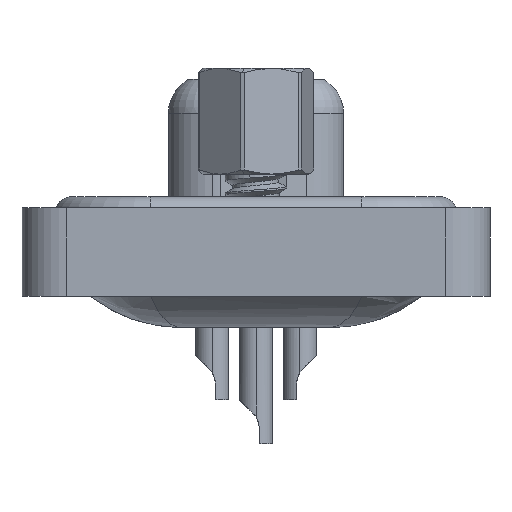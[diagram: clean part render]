
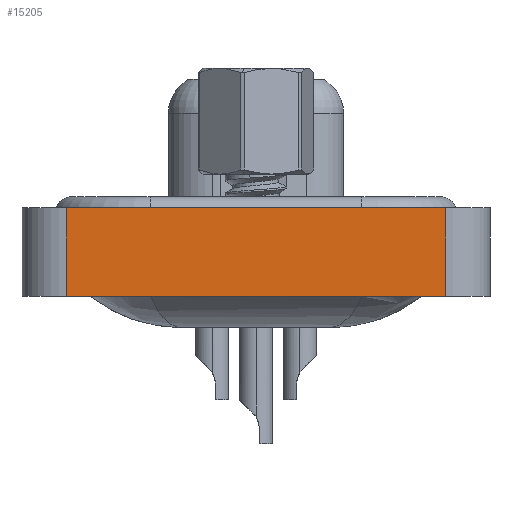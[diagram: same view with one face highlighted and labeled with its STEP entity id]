
A CAD part, left-side view. The second image highlights one B-rep face of the part: STEP entity #15205.
In plain terms, the highlighted planar face has unit normal (-1, 0, 0).
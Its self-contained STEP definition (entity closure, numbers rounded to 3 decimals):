
#445 = VERTEX_POINT ( 'NONE', #22338 ) ;
#742 = CARTESIAN_POINT ( 'NONE',  ( -7.26, -8.55, -3.6 ) ) ;
#1912 = VECTOR ( 'NONE', #21880, 1000. ) ;
#1967 = CARTESIAN_POINT ( 'NONE',  ( -7.26, 8.55, 0.4 ) ) ;
#2844 = LINE ( 'NONE', #4650, #15499 ) ;
#3188 = ORIENTED_EDGE ( 'NONE', *, *, #18547, .T. ) ;
#4125 = ORIENTED_EDGE ( 'NONE', *, *, #7252, .F. ) ;
#4650 = CARTESIAN_POINT ( 'NONE',  ( -7.26, -8.55, 0.4 ) ) ;
#6713 = LINE ( 'NONE', #12430, #25580 ) ;
#7168 = DIRECTION ( 'NONE',  ( 0., 0., 1. ) ) ;
#7252 = EDGE_CURVE ( 'NONE', #19398, #445, #2844, .T. ) ;
#7758 = VERTEX_POINT ( 'NONE', #742 ) ;
#10339 = EDGE_CURVE ( 'NONE', #7758, #445, #6713, .T. ) ;
#10732 = EDGE_LOOP ( 'NONE', ( #25264, #4125, #11559, #3188 ) ) ;
#11206 = FACE_OUTER_BOUND ( 'NONE', #10732, .T. ) ;
#11559 = ORIENTED_EDGE ( 'NONE', *, *, #23377, .F. ) ;
#12430 = CARTESIAN_POINT ( 'NONE',  ( -7.26, -8.55, -3.6 ) ) ;
#12632 = CARTESIAN_POINT ( 'NONE',  ( -7.26, -8.55, -3.6 ) ) ;
#12662 = CARTESIAN_POINT ( 'NONE',  ( -7.26, 8.55, -3.6 ) ) ;
#13392 = DIRECTION ( 'NONE',  ( -1., 0., 0. ) ) ;
#13637 = VECTOR ( 'NONE', #20549, 1000. ) ;
#14175 = VERTEX_POINT ( 'NONE', #12662 ) ;
#14718 = LINE ( 'NONE', #12632, #13637 ) ;
#15205 = ADVANCED_FACE ( 'NONE', ( #11206 ), #15231, .T. ) ;
#15231 = PLANE ( 'NONE',  #19509 ) ;
#15499 = VECTOR ( 'NONE', #18659, 1000. ) ;
#18409 = DIRECTION ( 'NONE',  ( 0., 0., 1. ) ) ;
#18547 = EDGE_CURVE ( 'NONE', #14175, #7758, #14718, .T. ) ;
#18659 = DIRECTION ( 'NONE',  ( 0., -1., 0. ) ) ;
#19398 = VERTEX_POINT ( 'NONE', #1967 ) ;
#19509 = AXIS2_PLACEMENT_3D ( 'NONE', #23118, #13392, #7168 ) ;
#19824 = LINE ( 'NONE', #23836, #1912 ) ;
#20549 = DIRECTION ( 'NONE',  ( 0., -1., 0. ) ) ;
#21880 = DIRECTION ( 'NONE',  ( 0., 0., 1. ) ) ;
#22338 = CARTESIAN_POINT ( 'NONE',  ( -7.26, -8.55, 0.4 ) ) ;
#23118 = CARTESIAN_POINT ( 'NONE',  ( -7.26, -8.55, -3.6 ) ) ;
#23377 = EDGE_CURVE ( 'NONE', #14175, #19398, #19824, .T. ) ;
#23836 = CARTESIAN_POINT ( 'NONE',  ( -7.26, 8.55, -3.6 ) ) ;
#25264 = ORIENTED_EDGE ( 'NONE', *, *, #10339, .T. ) ;
#25580 = VECTOR ( 'NONE', #18409, 1000. ) ;
